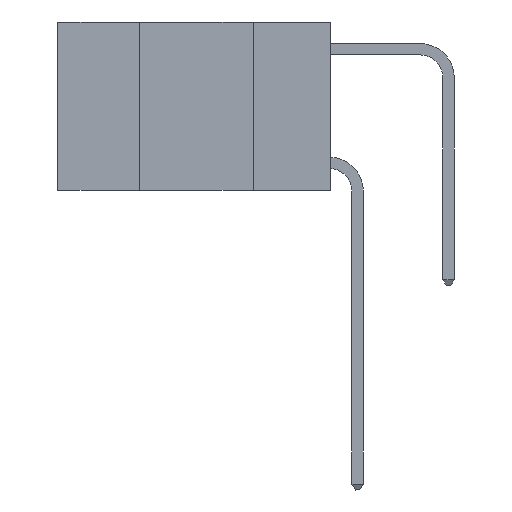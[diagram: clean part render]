
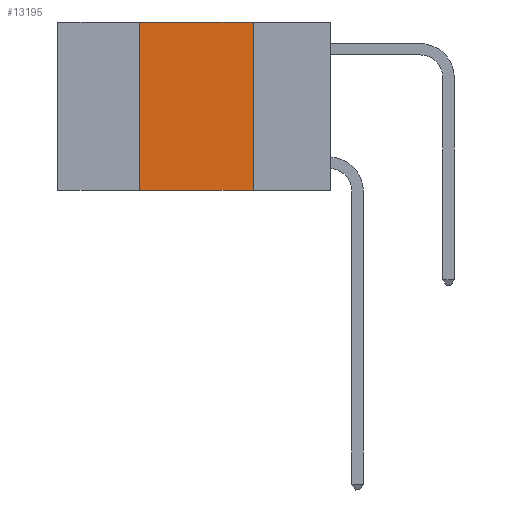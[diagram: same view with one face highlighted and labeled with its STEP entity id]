
A CAD part, left-side view. The second image highlights one B-rep face of the part: STEP entity #13195.
In plain terms, the highlighted planar face has unit normal (-1, 0, 0).
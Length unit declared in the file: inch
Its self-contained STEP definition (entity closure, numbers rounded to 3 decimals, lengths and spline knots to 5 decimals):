
#244 = CARTESIAN_POINT ( 'NONE',  ( 0., 0.42, 0. ) ) ;
#635 = LINE ( 'NONE', #8140, #9381 ) ;
#857 = VECTOR ( 'NONE', #6194, 39.37008 ) ;
#1035 = CARTESIAN_POINT ( 'NONE',  ( 0., 0.6, -0.37 ) ) ;
#1247 = DIRECTION ( 'NONE',  ( 0., -1., 0. ) ) ;
#1476 = VERTEX_POINT ( 'NONE', #12052 ) ;
#2210 = DIRECTION ( 'NONE',  ( 0., 0., -1. ) ) ;
#2714 = CARTESIAN_POINT ( 'NONE',  ( 0., 0.17, -0.37 ) ) ;
#3040 = EDGE_LOOP ( 'NONE', ( #8121, #10775, #11290, #10729 ) ) ;
#3271 = VERTEX_POINT ( 'NONE', #12097 ) ;
#3272 = LINE ( 'NONE', #244, #857 ) ;
#3686 = LINE ( 'NONE', #1035, #10752 ) ;
#3826 = VERTEX_POINT ( 'NONE', #12090 ) ;
#5936 = DIRECTION ( 'NONE',  ( 0., -1., 0. ) ) ;
#5994 = PLANE ( 'NONE',  #12965 ) ;
#6172 = LINE ( 'NONE', #13172, #6362 ) ;
#6194 = DIRECTION ( 'NONE',  ( 0., 0., 1. ) ) ;
#6362 = VECTOR ( 'NONE', #1247, 39.37008 ) ;
#6380 = EDGE_CURVE ( 'NONE', #3826, #8512, #635, .T. ) ;
#7297 = EDGE_CURVE ( 'NONE', #1476, #3826, #6172, .T. ) ;
#7831 = FACE_OUTER_BOUND ( 'NONE', #3040, .T. ) ;
#8121 = ORIENTED_EDGE ( 'NONE', *, *, #6380, .F. ) ;
#8140 = CARTESIAN_POINT ( 'NONE',  ( 0., 0.17, 0. ) ) ;
#8447 = DIRECTION ( 'NONE',  ( 0., 0., -1. ) ) ;
#8512 = VERTEX_POINT ( 'NONE', #2714 ) ;
#8998 = EDGE_CURVE ( 'NONE', #3271, #8512, #3686, .T. ) ;
#9381 = VECTOR ( 'NONE', #2210, 39.37008 ) ;
#9573 = CARTESIAN_POINT ( 'NONE',  ( 0., 0.6, 0. ) ) ;
#10174 = EDGE_CURVE ( 'NONE', #3271, #1476, #3272, .T. ) ;
#10729 = ORIENTED_EDGE ( 'NONE', *, *, #8998, .T. ) ;
#10752 = VECTOR ( 'NONE', #5936, 39.37008 ) ;
#10771 = DIRECTION ( 'NONE',  ( 1., 0., 0. ) ) ;
#10775 = ORIENTED_EDGE ( 'NONE', *, *, #7297, .F. ) ;
#11290 = ORIENTED_EDGE ( 'NONE', *, *, #10174, .F. ) ;
#12052 = CARTESIAN_POINT ( 'NONE',  ( 0., 0.42, 0. ) ) ;
#12090 = CARTESIAN_POINT ( 'NONE',  ( 0., 0.17, 0. ) ) ;
#12097 = CARTESIAN_POINT ( 'NONE',  ( 0., 0.42, -0.37 ) ) ;
#12965 = AXIS2_PLACEMENT_3D ( 'NONE', #9573, #10771, #8447 ) ;
#13172 = CARTESIAN_POINT ( 'NONE',  ( 0., 0.6, 0. ) ) ;
#13195 = ADVANCED_FACE ( 'NONE', ( #7831 ), #5994, .F. ) ;
